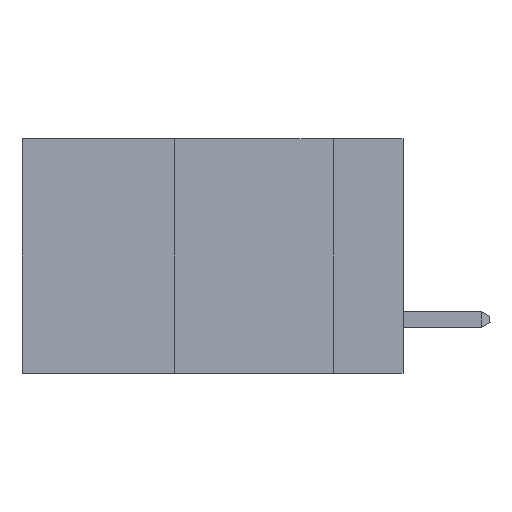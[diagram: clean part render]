
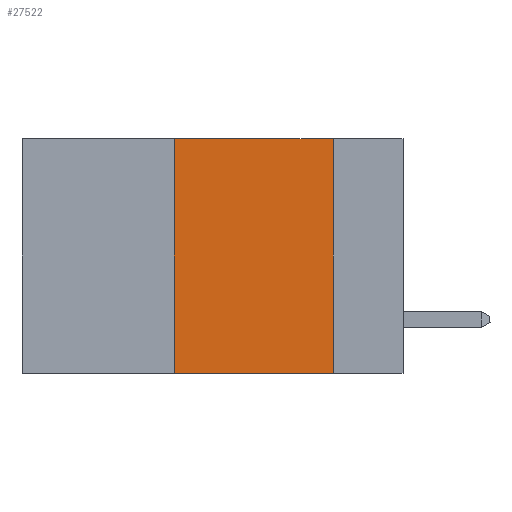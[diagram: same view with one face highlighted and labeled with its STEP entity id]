
A CAD part, left-side view. The second image highlights one B-rep face of the part: STEP entity #27522.
In plain terms, the highlighted planar face has unit normal (-1, 0, 0).
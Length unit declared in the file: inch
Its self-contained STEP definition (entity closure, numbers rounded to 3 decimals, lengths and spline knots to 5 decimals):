
#88 = CARTESIAN_POINT ( 'NONE',  ( 0., 0.36, 0. ) ) ;
#929 = LINE ( 'NONE', #2386, #21980 ) ;
#1488 = ORIENTED_EDGE ( 'NONE', *, *, #26344, .F. ) ;
#1563 = ORIENTED_EDGE ( 'NONE', *, *, #27907, .F. ) ;
#1840 = DIRECTION ( 'NONE',  ( 1., 0., 0. ) ) ;
#2302 = EDGE_CURVE ( 'NONE', #28982, #29406, #14415, .T. ) ;
#2386 = CARTESIAN_POINT ( 'NONE',  ( 0., 0.36, 0. ) ) ;
#6180 = ORIENTED_EDGE ( 'NONE', *, *, #2302, .F. ) ;
#6378 = ORIENTED_EDGE ( 'NONE', *, *, #27032, .T. ) ;
#6774 = AXIS2_PLACEMENT_3D ( 'NONE', #23984, #1840, #21751 ) ;
#9680 = CARTESIAN_POINT ( 'NONE',  ( 0., 0.6, 0. ) ) ;
#10154 = VECTOR ( 'NONE', #28698, 39.37008 ) ;
#13980 = VERTEX_POINT ( 'NONE', #88 ) ;
#14415 = LINE ( 'NONE', #15970, #10154 ) ;
#15695 = CARTESIAN_POINT ( 'NONE',  ( 0., 0.36, -0.37 ) ) ;
#15970 = CARTESIAN_POINT ( 'NONE',  ( 0., 0.11, 0. ) ) ;
#18570 = PLANE ( 'NONE',  #6774 ) ;
#19678 = DIRECTION ( 'NONE',  ( 0., 0., 1. ) ) ;
#20813 = VECTOR ( 'NONE', #29403, 39.37008 ) ;
#21219 = LINE ( 'NONE', #26993, #20813 ) ;
#21751 = DIRECTION ( 'NONE',  ( 0., 0., -1. ) ) ;
#21980 = VECTOR ( 'NONE', #19678, 39.37008 ) ;
#23860 = VERTEX_POINT ( 'NONE', #15695 ) ;
#23984 = CARTESIAN_POINT ( 'NONE',  ( 0., 0.6, 0. ) ) ;
#24151 = LINE ( 'NONE', #9680, #28021 ) ;
#24378 = EDGE_LOOP ( 'NONE', ( #6180, #1563, #1488, #6378 ) ) ;
#24543 = FACE_OUTER_BOUND ( 'NONE', #24378, .T. ) ;
#26344 = EDGE_CURVE ( 'NONE', #23860, #13980, #929, .T. ) ;
#26653 = CARTESIAN_POINT ( 'NONE',  ( 0., 0.11, 0. ) ) ;
#26782 = DIRECTION ( 'NONE',  ( 0., -1., 0. ) ) ;
#26993 = CARTESIAN_POINT ( 'NONE',  ( 0., 0.6, -0.37 ) ) ;
#27032 = EDGE_CURVE ( 'NONE', #23860, #29406, #21219, .T. ) ;
#27522 = ADVANCED_FACE ( 'NONE', ( #24543 ), #18570, .F. ) ;
#27907 = EDGE_CURVE ( 'NONE', #13980, #28982, #24151, .T. ) ;
#28021 = VECTOR ( 'NONE', #26782, 39.37008 ) ;
#28698 = DIRECTION ( 'NONE',  ( 0., 0., -1. ) ) ;
#28982 = VERTEX_POINT ( 'NONE', #26653 ) ;
#29403 = DIRECTION ( 'NONE',  ( 0., -1., 0. ) ) ;
#29406 = VERTEX_POINT ( 'NONE', #30640 ) ;
#30640 = CARTESIAN_POINT ( 'NONE',  ( 0., 0.11, -0.37 ) ) ;
